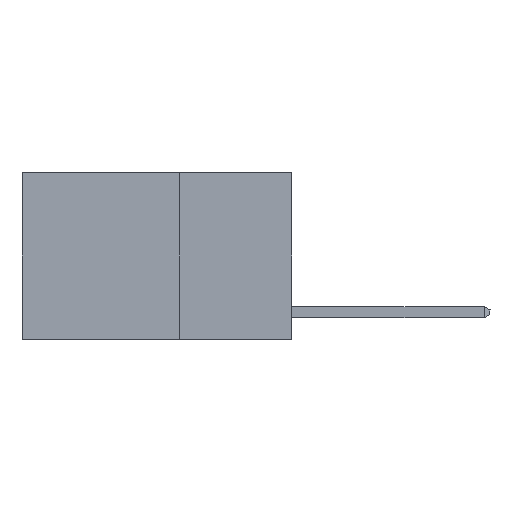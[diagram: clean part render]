
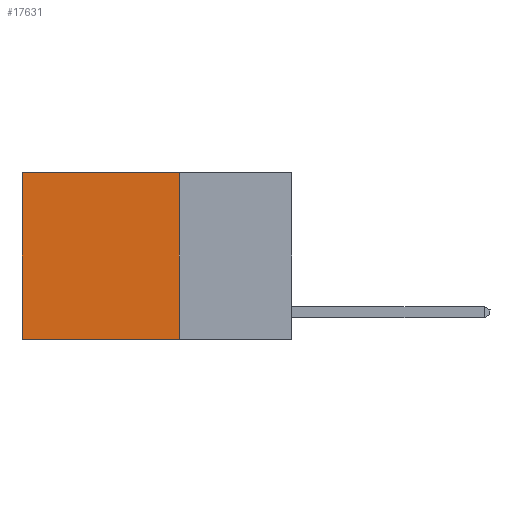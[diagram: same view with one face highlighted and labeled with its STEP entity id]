
A CAD part, left-side view. The second image highlights one B-rep face of the part: STEP entity #17631.
In plain terms, the highlighted planar face has unit normal (-1, 0, 0).
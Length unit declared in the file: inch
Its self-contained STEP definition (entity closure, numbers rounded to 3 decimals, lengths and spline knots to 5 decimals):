
#771 = ORIENTED_EDGE ( 'NONE', *, *, #23065, .T. ) ;
#2662 = DIRECTION ( 'NONE',  ( 1., 0., 0. ) ) ;
#2870 = VECTOR ( 'NONE', #22742, 39.37008 ) ;
#3573 = CARTESIAN_POINT ( 'NONE',  ( 0.2625, 0.6, -0.37 ) ) ;
#4345 = DIRECTION ( 'NONE',  ( 0., 0., -1. ) ) ;
#5611 = VECTOR ( 'NONE', #24280, 39.37008 ) ;
#5909 = EDGE_LOOP ( 'NONE', ( #771, #18871, #21243, #10845 ) ) ;
#6744 = CARTESIAN_POINT ( 'NONE',  ( 0.2625, 0.25, -0.37 ) ) ;
#6898 = LINE ( 'NONE', #17914, #23106 ) ;
#8553 = CARTESIAN_POINT ( 'NONE',  ( 0.2625, 0.25, 0. ) ) ;
#8638 = CARTESIAN_POINT ( 'NONE',  ( 0.2625, 0.25, 0. ) ) ;
#9242 = LINE ( 'NONE', #9637, #10438 ) ;
#9307 = LINE ( 'NONE', #6744, #2870 ) ;
#9543 = DIRECTION ( 'NONE',  ( 0., 1., 0. ) ) ;
#9637 = CARTESIAN_POINT ( 'NONE',  ( 0.2625, 0.25, 0. ) ) ;
#10438 = VECTOR ( 'NONE', #9543, 39.37008 ) ;
#10845 = ORIENTED_EDGE ( 'NONE', *, *, #13188, .T. ) ;
#12228 = VERTEX_POINT ( 'NONE', #18450 ) ;
#13162 = VERTEX_POINT ( 'NONE', #3573 ) ;
#13188 = EDGE_CURVE ( 'NONE', #15194, #24042, #9242, .T. ) ;
#14471 = CARTESIAN_POINT ( 'NONE',  ( 0.2625, 0.25, 0. ) ) ;
#15194 = VERTEX_POINT ( 'NONE', #14471 ) ;
#17631 = ADVANCED_FACE ( 'NONE', ( #24937 ), #18048, .F. ) ;
#17862 = CARTESIAN_POINT ( 'NONE',  ( 0.2625, 0.6, 0. ) ) ;
#17914 = CARTESIAN_POINT ( 'NONE',  ( 0.2625, 0.6, 0. ) ) ;
#18048 = PLANE ( 'NONE',  #23569 ) ;
#18450 = CARTESIAN_POINT ( 'NONE',  ( 0.2625, 0.25, -0.37 ) ) ;
#18871 = ORIENTED_EDGE ( 'NONE', *, *, #23683, .F. ) ;
#21243 = ORIENTED_EDGE ( 'NONE', *, *, #24302, .F. ) ;
#21802 = LINE ( 'NONE', #8638, #5611 ) ;
#22742 = DIRECTION ( 'NONE',  ( 0., 1., 0. ) ) ;
#23065 = EDGE_CURVE ( 'NONE', #24042, #13162, #6898, .T. ) ;
#23106 = VECTOR ( 'NONE', #4345, 39.37008 ) ;
#23569 = AXIS2_PLACEMENT_3D ( 'NONE', #8553, #2662, #24021 ) ;
#23683 = EDGE_CURVE ( 'NONE', #12228, #13162, #9307, .T. ) ;
#24021 = DIRECTION ( 'NONE',  ( 0., 0., -1. ) ) ;
#24042 = VERTEX_POINT ( 'NONE', #17862 ) ;
#24280 = DIRECTION ( 'NONE',  ( 0., 0., -1. ) ) ;
#24302 = EDGE_CURVE ( 'NONE', #15194, #12228, #21802, .T. ) ;
#24937 = FACE_OUTER_BOUND ( 'NONE', #5909, .T. ) ;
